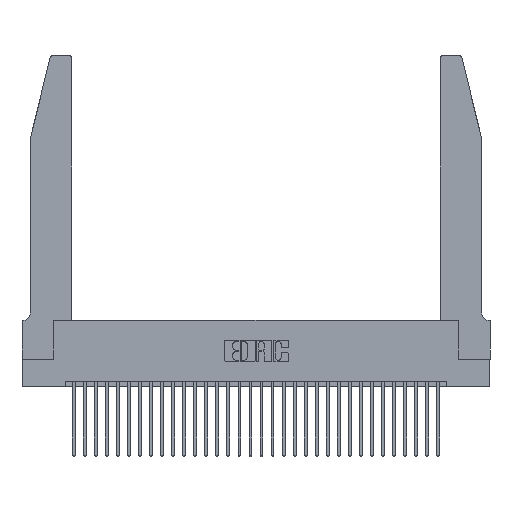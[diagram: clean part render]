
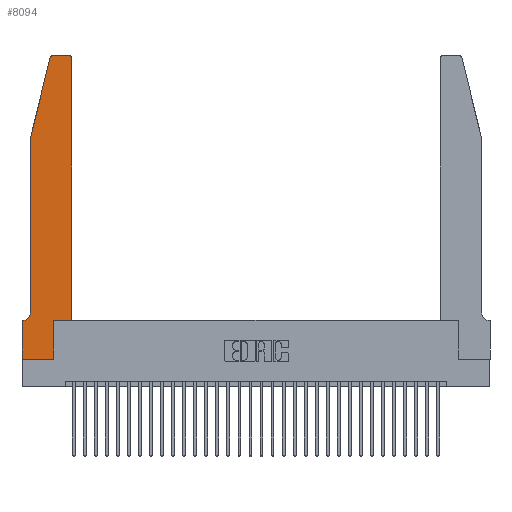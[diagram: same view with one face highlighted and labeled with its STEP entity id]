
A CAD part, top view. The second image highlights one B-rep face of the part: STEP entity #8094.
In plain terms, the highlighted planar face has unit normal (0, 0, 1).
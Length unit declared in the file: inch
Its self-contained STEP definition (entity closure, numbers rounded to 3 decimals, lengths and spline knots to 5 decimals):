
#10 = EDGE_CURVE ( 'NONE', #31387, #30597, #7170, .T. ) ;
#242 = EDGE_CURVE ( 'NONE', #25407, #8420, #4393, .T. ) ;
#314 = EDGE_CURVE ( 'NONE', #12832, #10154, #21698, .T. ) ;
#322 = ORIENTED_EDGE ( 'NONE', *, *, #24142, .T. ) ;
#1147 = EDGE_CURVE ( 'NONE', #10154, #23003, #30261, .T. ) ;
#1823 = EDGE_CURVE ( 'NONE', #13740, #27852, #8373, .T. ) ;
#1867 = PLANE ( 'NONE',  #5832 ) ;
#2138 = DIRECTION ( 'NONE',  ( -1., 0., 0. ) ) ;
#3046 = CIRCLE ( 'NONE', #16005, 0.07 ) ;
#3474 = VECTOR ( 'NONE', #9427, 39.37008 ) ;
#3978 = CARTESIAN_POINT ( 'NONE',  ( 0.0755, 2., 0.37 ) ) ;
#4259 = CARTESIAN_POINT ( 'NONE',  ( 0.284, 2.72, 0.37 ) ) ;
#4393 = LINE ( 'NONE', #15439, #23658 ) ;
#5444 = ORIENTED_EDGE ( 'NONE', *, *, #12694, .T. ) ;
#5832 = AXIS2_PLACEMENT_3D ( 'NONE', #31743, #20595, #25617 ) ;
#6247 = CIRCLE ( 'NONE', #29085, 0.03 ) ;
#6400 = VERTEX_POINT ( 'NONE', #10256 ) ;
#6641 = ORIENTED_EDGE ( 'NONE', *, *, #242, .T. ) ;
#7015 = EDGE_LOOP ( 'NONE', ( #31429, #322, #15381, #22750, #13130, #6641, #25663, #7904, #7373, #18183, #16435, #5444 ) ) ;
#7170 = LINE ( 'NONE', #3978, #19743 ) ;
#7373 = ORIENTED_EDGE ( 'NONE', *, *, #1147, .T. ) ;
#7417 = DIRECTION ( 'NONE',  ( -1., 0., 0. ) ) ;
#7904 = ORIENTED_EDGE ( 'NONE', *, *, #314, .T. ) ;
#8094 = ADVANCED_FACE ( 'NONE', ( #21872 ), #1867, .T. ) ;
#8373 = LINE ( 'NONE', #22005, #30039 ) ;
#8420 = VERTEX_POINT ( 'NONE', #19659 ) ;
#9295 = DIRECTION ( 'NONE',  ( 1., 0., 0. ) ) ;
#9427 = DIRECTION ( 'NONE',  ( 0., -1., 0. ) ) ;
#9620 = CARTESIAN_POINT ( 'NONE',  ( 0., 0., 0.37 ) ) ;
#9850 = DIRECTION ( 'NONE',  ( -1., 0., 0. ) ) ;
#10154 = VERTEX_POINT ( 'NONE', #10626 ) ;
#10256 = CARTESIAN_POINT ( 'NONE',  ( 0.4205, 2.75, 0.37 ) ) ;
#10288 = DIRECTION ( 'NONE',  ( 1., 0., 0. ) ) ;
#10307 = VECTOR ( 'NONE', #10288, 39.37008 ) ;
#10329 = CARTESIAN_POINT ( 'NONE',  ( 0.4505, 2.72, 0.37 ) ) ;
#10626 = CARTESIAN_POINT ( 'NONE',  ( 0.2865, 0., 0.37 ) ) ;
#10810 = VERTEX_POINT ( 'NONE', #29338 ) ;
#11349 = VECTOR ( 'NONE', #9850, 39.37008 ) ;
#12694 = EDGE_CURVE ( 'NONE', #27852, #6400, #23197, .T. ) ;
#12832 = VERTEX_POINT ( 'NONE', #22249 ) ;
#13130 = ORIENTED_EDGE ( 'NONE', *, *, #24763, .T. ) ;
#13585 = CARTESIAN_POINT ( 'NONE',  ( 0.0055, 0.35, 0.37 ) ) ;
#13740 = VERTEX_POINT ( 'NONE', #23621 ) ;
#13957 = EDGE_CURVE ( 'NONE', #8420, #12832, #15254, .T. ) ;
#14244 = VECTOR ( 'NONE', #28069, 39.37008 ) ;
#14581 = DIRECTION ( 'NONE',  ( 0., 1., 0. ) ) ;
#14624 = CARTESIAN_POINT ( 'NONE',  ( 0.2605, 2.75, 0.37 ) ) ;
#14715 = CARTESIAN_POINT ( 'NONE',  ( 0.4205, 2.72, 0.37 ) ) ;
#14868 = VECTOR ( 'NONE', #29668, 39.37008 ) ;
#14873 = LINE ( 'NONE', #19006, #3474 ) ;
#15254 = LINE ( 'NONE', #9620, #14868 ) ;
#15320 = VECTOR ( 'NONE', #14581, 39.37008 ) ;
#15381 = ORIENTED_EDGE ( 'NONE', *, *, #10, .T. ) ;
#15439 = CARTESIAN_POINT ( 'NONE',  ( 0.0755, 0.35, 0.37 ) ) ;
#15640 = CARTESIAN_POINT ( 'NONE',  ( 0., 0., 0.37 ) ) ;
#16005 = AXIS2_PLACEMENT_3D ( 'NONE', #32137, #29825, #2138 ) ;
#16022 = CARTESIAN_POINT ( 'NONE',  ( 0.284, 2.75, 0.37 ) ) ;
#16435 = ORIENTED_EDGE ( 'NONE', *, *, #1823, .T. ) ;
#17510 = CARTESIAN_POINT ( 'NONE',  ( 0.2865, 0.35, 0.37 ) ) ;
#18142 = EDGE_CURVE ( 'NONE', #6400, #21556, #25543, .T. ) ;
#18183 = ORIENTED_EDGE ( 'NONE', *, *, #21489, .T. ) ;
#19006 = CARTESIAN_POINT ( 'NONE',  ( 0.0755, 2., 0.37 ) ) ;
#19389 = EDGE_CURVE ( 'NONE', #30597, #10810, #14873, .T. ) ;
#19659 = CARTESIAN_POINT ( 'NONE',  ( 0., 0.35, 0.37 ) ) ;
#19743 = VECTOR ( 'NONE', #27321, 39.37008 ) ;
#20595 = DIRECTION ( 'NONE',  ( 0., 0., 1. ) ) ;
#21489 = EDGE_CURVE ( 'NONE', #23003, #13740, #30747, .T. ) ;
#21556 = VERTEX_POINT ( 'NONE', #16022 ) ;
#21698 = LINE ( 'NONE', #15640, #14244 ) ;
#21872 = FACE_OUTER_BOUND ( 'NONE', #7015, .T. ) ;
#22005 = CARTESIAN_POINT ( 'NONE',  ( 0.4505, 0.35, 0.37 ) ) ;
#22128 = DIRECTION ( 'NONE',  ( 0., 1., 0. ) ) ;
#22249 = CARTESIAN_POINT ( 'NONE',  ( 0., 0., 0.37 ) ) ;
#22750 = ORIENTED_EDGE ( 'NONE', *, *, #19389, .T. ) ;
#22842 = CARTESIAN_POINT ( 'NONE',  ( 0.4505, 0.35, 0.37 ) ) ;
#23003 = VERTEX_POINT ( 'NONE', #32130 ) ;
#23197 = CIRCLE ( 'NONE', #27443, 0.03 ) ;
#23621 = CARTESIAN_POINT ( 'NONE',  ( 0.4505, 0.35, 0.37 ) ) ;
#23658 = VECTOR ( 'NONE', #7417, 39.37008 ) ;
#24142 = EDGE_CURVE ( 'NONE', #21556, #31387, #6247, .T. ) ;
#24763 = EDGE_CURVE ( 'NONE', #10810, #25407, #3046, .T. ) ;
#25407 = VERTEX_POINT ( 'NONE', #13585 ) ;
#25543 = LINE ( 'NONE', #14624, #11349 ) ;
#25617 = DIRECTION ( 'NONE',  ( 1., 0., 0. ) ) ;
#25663 = ORIENTED_EDGE ( 'NONE', *, *, #13957, .T. ) ;
#27321 = DIRECTION ( 'NONE',  ( -0.239, -0.971, 0. ) ) ;
#27443 = AXIS2_PLACEMENT_3D ( 'NONE', #14715, #27662, #30179 ) ;
#27662 = DIRECTION ( 'NONE',  ( 0., 0., 1. ) ) ;
#27852 = VERTEX_POINT ( 'NONE', #10329 ) ;
#28069 = DIRECTION ( 'NONE',  ( 1., 0., 0. ) ) ;
#28300 = CARTESIAN_POINT ( 'NONE',  ( 0.0755, 2., 0.37 ) ) ;
#29085 = AXIS2_PLACEMENT_3D ( 'NONE', #4259, #29662, #9295 ) ;
#29338 = CARTESIAN_POINT ( 'NONE',  ( 0.0755, 0.42, 0.37 ) ) ;
#29662 = DIRECTION ( 'NONE',  ( 0., 0., 1. ) ) ;
#29668 = DIRECTION ( 'NONE',  ( 0., -1., 0. ) ) ;
#29825 = DIRECTION ( 'NONE',  ( 0., 0., -1. ) ) ;
#30039 = VECTOR ( 'NONE', #22128, 39.37008 ) ;
#30179 = DIRECTION ( 'NONE',  ( 1., 0., 0. ) ) ;
#30261 = LINE ( 'NONE', #17510, #15320 ) ;
#30582 = CARTESIAN_POINT ( 'NONE',  ( 0.25487, 2.72718, 0.37 ) ) ;
#30597 = VERTEX_POINT ( 'NONE', #28300 ) ;
#30747 = LINE ( 'NONE', #22842, #10307 ) ;
#31387 = VERTEX_POINT ( 'NONE', #30582 ) ;
#31429 = ORIENTED_EDGE ( 'NONE', *, *, #18142, .T. ) ;
#31743 = CARTESIAN_POINT ( 'NONE',  ( 0., 0.35, 0.37 ) ) ;
#32130 = CARTESIAN_POINT ( 'NONE',  ( 0.2865, 0.35, 0.37 ) ) ;
#32137 = CARTESIAN_POINT ( 'NONE',  ( 0.0055, 0.42, 0.37 ) ) ;
